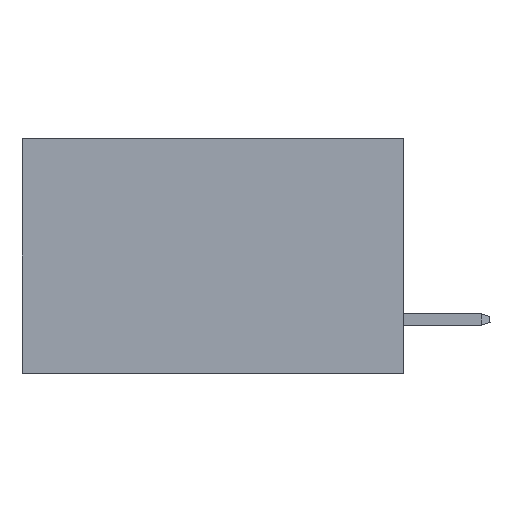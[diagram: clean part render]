
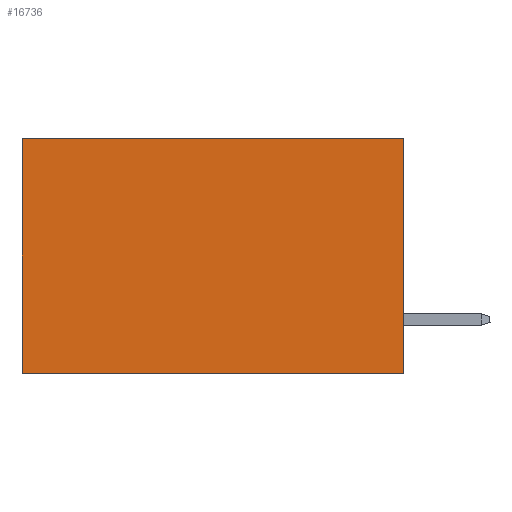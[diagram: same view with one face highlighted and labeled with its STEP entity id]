
A CAD part, left-side view. The second image highlights one B-rep face of the part: STEP entity #16736.
In plain terms, the highlighted planar face has unit normal (-1, 0, 0).
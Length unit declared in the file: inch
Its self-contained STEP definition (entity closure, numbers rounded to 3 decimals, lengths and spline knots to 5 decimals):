
#2941 = CARTESIAN_POINT ( 'NONE',  ( 0.2875, 0.6, 0. ) ) ;
#3171 = EDGE_CURVE ( 'NONE', #33629, #7960, #36135, .T. ) ;
#3396 = FACE_OUTER_BOUND ( 'NONE', #7275, .T. ) ;
#5329 = VECTOR ( 'NONE', #27871, 39.37008 ) ;
#6230 = DIRECTION ( 'NONE',  ( 1., 0., 0. ) ) ;
#7275 = EDGE_LOOP ( 'NONE', ( #19844, #10077, #23059, #13445 ) ) ;
#7621 = EDGE_CURVE ( 'NONE', #31909, #33629, #39413, .T. ) ;
#7960 = VERTEX_POINT ( 'NONE', #29844 ) ;
#8375 = CARTESIAN_POINT ( 'NONE',  ( 0.2875, 0., -0.37 ) ) ;
#8491 = CARTESIAN_POINT ( 'NONE',  ( 0.2875, 0., 0. ) ) ;
#9894 = PLANE ( 'NONE',  #33940 ) ;
#10077 = ORIENTED_EDGE ( 'NONE', *, *, #3171, .F. ) ;
#11646 = CARTESIAN_POINT ( 'NONE',  ( 0.2875, 0., 0. ) ) ;
#12562 = LINE ( 'NONE', #15400, #13589 ) ;
#13150 = EDGE_CURVE ( 'NONE', #32689, #7960, #15130, .T. ) ;
#13445 = ORIENTED_EDGE ( 'NONE', *, *, #34764, .T. ) ;
#13589 = VECTOR ( 'NONE', #24921, 39.37008 ) ;
#15130 = LINE ( 'NONE', #2941, #5329 ) ;
#15400 = CARTESIAN_POINT ( 'NONE',  ( 0.2875, 0., 0. ) ) ;
#15772 = VECTOR ( 'NONE', #33335, 39.37008 ) ;
#16736 = ADVANCED_FACE ( 'NONE', ( #3396 ), #9894, .F. ) ;
#19019 = DIRECTION ( 'NONE',  ( 0., 0., -1. ) ) ;
#19213 = CARTESIAN_POINT ( 'NONE',  ( 0.2875, 0., 0. ) ) ;
#19844 = ORIENTED_EDGE ( 'NONE', *, *, #13150, .T. ) ;
#20414 = CARTESIAN_POINT ( 'NONE',  ( 0.2875, 0., -0.37 ) ) ;
#23059 = ORIENTED_EDGE ( 'NONE', *, *, #7621, .F. ) ;
#24921 = DIRECTION ( 'NONE',  ( 0., 1., 0. ) ) ;
#27871 = DIRECTION ( 'NONE',  ( 0., 0., -1. ) ) ;
#29844 = CARTESIAN_POINT ( 'NONE',  ( 0.2875, 0.6, -0.37 ) ) ;
#29893 = DIRECTION ( 'NONE',  ( 0., 0., -1. ) ) ;
#31909 = VERTEX_POINT ( 'NONE', #8491 ) ;
#32500 = CARTESIAN_POINT ( 'NONE',  ( 0.2875, 0.6, 0. ) ) ;
#32689 = VERTEX_POINT ( 'NONE', #32500 ) ;
#33335 = DIRECTION ( 'NONE',  ( 0., 1., 0. ) ) ;
#33629 = VERTEX_POINT ( 'NONE', #20414 ) ;
#33940 = AXIS2_PLACEMENT_3D ( 'NONE', #19213, #6230, #19019 ) ;
#34304 = VECTOR ( 'NONE', #29893, 39.37008 ) ;
#34764 = EDGE_CURVE ( 'NONE', #31909, #32689, #12562, .T. ) ;
#36135 = LINE ( 'NONE', #8375, #15772 ) ;
#39413 = LINE ( 'NONE', #11646, #34304 ) ;
